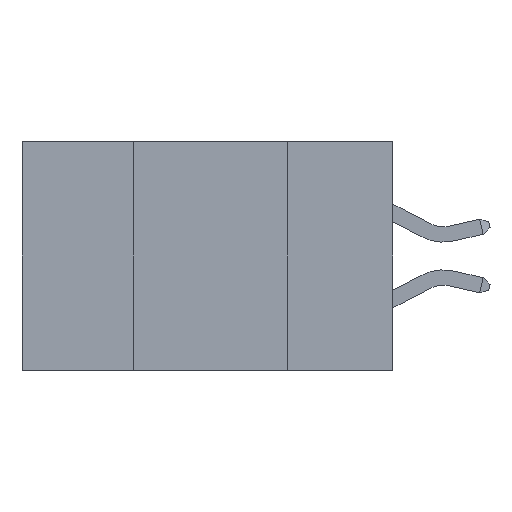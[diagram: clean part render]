
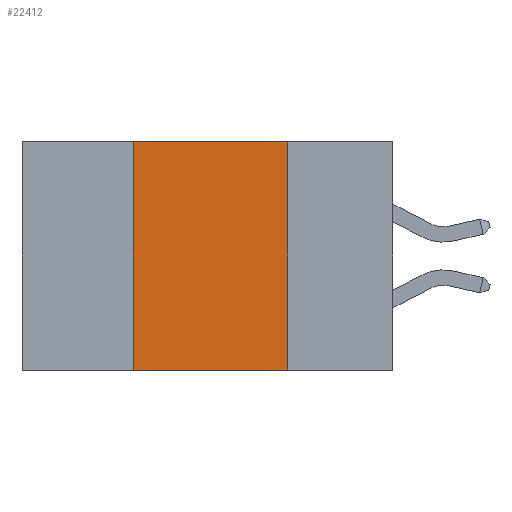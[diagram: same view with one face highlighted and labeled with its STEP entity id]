
A CAD part, left-side view. The second image highlights one B-rep face of the part: STEP entity #22412.
In plain terms, the highlighted planar face has unit normal (-1, 0, 0).
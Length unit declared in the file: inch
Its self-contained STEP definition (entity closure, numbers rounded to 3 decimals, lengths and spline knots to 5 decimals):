
#1094 = PLANE ( 'NONE',  #30518 ) ;
#2193 = CARTESIAN_POINT ( 'NONE',  ( 0., 0.42, -0.37 ) ) ;
#3556 = DIRECTION ( 'NONE',  ( 0., -1., 0. ) ) ;
#4921 = CARTESIAN_POINT ( 'NONE',  ( 0., 0.17, 0. ) ) ;
#6775 = VERTEX_POINT ( 'NONE', #2193 ) ;
#6816 = CARTESIAN_POINT ( 'NONE',  ( 0., 0.6, -0.37 ) ) ;
#8300 = DIRECTION ( 'NONE',  ( 0., 0., -1. ) ) ;
#9740 = LINE ( 'NONE', #32677, #26750 ) ;
#10293 = VERTEX_POINT ( 'NONE', #19152 ) ;
#11249 = CARTESIAN_POINT ( 'NONE',  ( 0., 0.6, 0. ) ) ;
#11255 = VERTEX_POINT ( 'NONE', #23824 ) ;
#11726 = ORIENTED_EDGE ( 'NONE', *, *, #36414, .F. ) ;
#13318 = ORIENTED_EDGE ( 'NONE', *, *, #40395, .F. ) ;
#14673 = DIRECTION ( 'NONE',  ( 0., 0., -1. ) ) ;
#15133 = LINE ( 'NONE', #6816, #32105 ) ;
#16980 = CARTESIAN_POINT ( 'NONE',  ( 0., 0.17, 0. ) ) ;
#19152 = CARTESIAN_POINT ( 'NONE',  ( 0., 0.42, 0. ) ) ;
#22412 = ADVANCED_FACE ( 'NONE', ( #40984 ), #1094, .F. ) ;
#22453 = DIRECTION ( 'NONE',  ( 0., -1., 0. ) ) ;
#22847 = LINE ( 'NONE', #4921, #40714 ) ;
#22871 = EDGE_CURVE ( 'NONE', #6775, #11255, #15133, .T. ) ;
#23048 = DIRECTION ( 'NONE',  ( 0., 0., 1. ) ) ;
#23824 = CARTESIAN_POINT ( 'NONE',  ( 0., 0.17, -0.37 ) ) ;
#24477 = VERTEX_POINT ( 'NONE', #16980 ) ;
#24507 = ORIENTED_EDGE ( 'NONE', *, *, #43161, .F. ) ;
#26750 = VECTOR ( 'NONE', #22453, 39.37008 ) ;
#27474 = EDGE_LOOP ( 'NONE', ( #13318, #24507, #11726, #28245 ) ) ;
#28245 = ORIENTED_EDGE ( 'NONE', *, *, #22871, .T. ) ;
#30518 = AXIS2_PLACEMENT_3D ( 'NONE', #11249, #34929, #14673 ) ;
#30606 = LINE ( 'NONE', #39779, #38389 ) ;
#32105 = VECTOR ( 'NONE', #3556, 39.37008 ) ;
#32677 = CARTESIAN_POINT ( 'NONE',  ( 0., 0.6, 0. ) ) ;
#34929 = DIRECTION ( 'NONE',  ( 1., 0., 0. ) ) ;
#36414 = EDGE_CURVE ( 'NONE', #6775, #10293, #30606, .T. ) ;
#38389 = VECTOR ( 'NONE', #23048, 39.37008 ) ;
#39779 = CARTESIAN_POINT ( 'NONE',  ( 0., 0.42, 0. ) ) ;
#40395 = EDGE_CURVE ( 'NONE', #24477, #11255, #22847, .T. ) ;
#40714 = VECTOR ( 'NONE', #8300, 39.37008 ) ;
#40984 = FACE_OUTER_BOUND ( 'NONE', #27474, .T. ) ;
#43161 = EDGE_CURVE ( 'NONE', #10293, #24477, #9740, .T. ) ;
